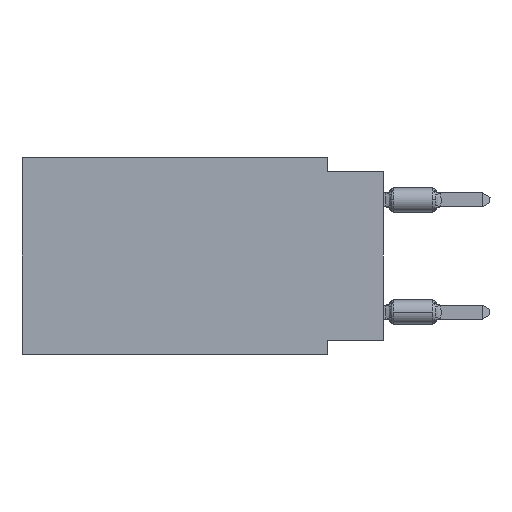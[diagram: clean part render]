
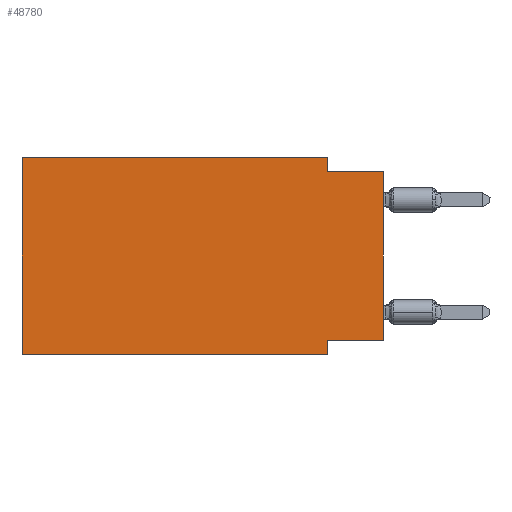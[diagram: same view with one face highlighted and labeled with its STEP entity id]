
A CAD part, left-side view. The second image highlights one B-rep face of the part: STEP entity #48780.
In plain terms, the highlighted planar face has unit normal (-1, 0, 0).
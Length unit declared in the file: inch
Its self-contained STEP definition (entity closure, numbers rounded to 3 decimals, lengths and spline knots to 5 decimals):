
#2103 = LINE ( 'NONE', #14832, #36640 ) ;
#2127 = EDGE_LOOP ( 'NONE', ( #13513, #40469, #35903, #5322, #4521, #36435, #36315, #18551 ) ) ;
#4039 = CARTESIAN_POINT ( 'NONE',  ( 0., 0.645, -0.35 ) ) ;
#4342 = FACE_OUTER_BOUND ( 'NONE', #2127, .T. ) ;
#4521 = ORIENTED_EDGE ( 'NONE', *, *, #28124, .F. ) ;
#5254 = CARTESIAN_POINT ( 'NONE',  ( 0., 0.1, -0.025 ) ) ;
#5322 = ORIENTED_EDGE ( 'NONE', *, *, #10600, .F. ) ;
#5991 = CARTESIAN_POINT ( 'NONE',  ( 0., 0.1, -0.35 ) ) ;
#7587 = LINE ( 'NONE', #23304, #27997 ) ;
#7668 = DIRECTION ( 'NONE',  ( 0., 0., -1. ) ) ;
#7987 = VERTEX_POINT ( 'NONE', #14603 ) ;
#10600 = EDGE_CURVE ( 'NONE', #7987, #50869, #49527, .T. ) ;
#10712 = EDGE_CURVE ( 'NONE', #32661, #44551, #46809, .T. ) ;
#11478 = CARTESIAN_POINT ( 'NONE',  ( 0., 0.1, -0.325 ) ) ;
#12235 = CARTESIAN_POINT ( 'NONE',  ( 0., 0.645, 0. ) ) ;
#13513 = ORIENTED_EDGE ( 'NONE', *, *, #34205, .T. ) ;
#14603 = CARTESIAN_POINT ( 'NONE',  ( 0., 0.645, 0. ) ) ;
#14832 = CARTESIAN_POINT ( 'NONE',  ( 0., 0.645, 0. ) ) ;
#16035 = EDGE_CURVE ( 'NONE', #44551, #33848, #43034, .T. ) ;
#16199 = AXIS2_PLACEMENT_3D ( 'NONE', #50549, #38377, #45419 ) ;
#16361 = VECTOR ( 'NONE', #24399, 39.37008 ) ;
#18551 = ORIENTED_EDGE ( 'NONE', *, *, #10712, .F. ) ;
#19239 = CARTESIAN_POINT ( 'NONE',  ( 0., 0., 0. ) ) ;
#20438 = CARTESIAN_POINT ( 'NONE',  ( 0., 0., -0.325 ) ) ;
#21376 = VERTEX_POINT ( 'NONE', #5254 ) ;
#22820 = CARTESIAN_POINT ( 'NONE',  ( 0., 0., -0.025 ) ) ;
#22997 = VECTOR ( 'NONE', #50339, 39.37008 ) ;
#23304 = CARTESIAN_POINT ( 'NONE',  ( 0., 0.645, -0.35 ) ) ;
#24399 = DIRECTION ( 'NONE',  ( 0., -1., 0. ) ) ;
#24421 = LINE ( 'NONE', #39720, #49111 ) ;
#24472 = VECTOR ( 'NONE', #7668, 39.37008 ) ;
#24663 = EDGE_CURVE ( 'NONE', #50869, #21376, #40655, .T. ) ;
#25563 = CARTESIAN_POINT ( 'NONE',  ( 0., 0.1, -0.35 ) ) ;
#26189 = DIRECTION ( 'NONE',  ( 0., 0., 1. ) ) ;
#27438 = VECTOR ( 'NONE', #28402, 39.37008 ) ;
#27997 = VECTOR ( 'NONE', #52208, 39.37008 ) ;
#28124 = EDGE_CURVE ( 'NONE', #50912, #7987, #2103, .T. ) ;
#28402 = DIRECTION ( 'NONE',  ( 0., 0., 1. ) ) ;
#32661 = VERTEX_POINT ( 'NONE', #20438 ) ;
#33848 = VERTEX_POINT ( 'NONE', #25563 ) ;
#34205 = EDGE_CURVE ( 'NONE', #32661, #48083, #35963, .T. ) ;
#35599 = EDGE_CURVE ( 'NONE', #21376, #48083, #24421, .T. ) ;
#35903 = ORIENTED_EDGE ( 'NONE', *, *, #24663, .F. ) ;
#35963 = LINE ( 'NONE', #19239, #27438 ) ;
#36315 = ORIENTED_EDGE ( 'NONE', *, *, #16035, .F. ) ;
#36435 = ORIENTED_EDGE ( 'NONE', *, *, #43540, .T. ) ;
#36640 = VECTOR ( 'NONE', #26189, 39.37008 ) ;
#38377 = DIRECTION ( 'NONE',  ( 1., 0., 0. ) ) ;
#39720 = CARTESIAN_POINT ( 'NONE',  ( 0., 0., -0.025 ) ) ;
#40388 = CARTESIAN_POINT ( 'NONE',  ( 0., 0.1, 0. ) ) ;
#40469 = ORIENTED_EDGE ( 'NONE', *, *, #35599, .F. ) ;
#40655 = LINE ( 'NONE', #40388, #24472 ) ;
#41641 = PLANE ( 'NONE',  #16199 ) ;
#42231 = DIRECTION ( 'NONE',  ( 0., 1., 0. ) ) ;
#42502 = CARTESIAN_POINT ( 'NONE',  ( 0., 0., -0.325 ) ) ;
#42553 = CARTESIAN_POINT ( 'NONE',  ( 0., 0.1, 0. ) ) ;
#43034 = LINE ( 'NONE', #5991, #22997 ) ;
#43540 = EDGE_CURVE ( 'NONE', #50912, #33848, #7587, .T. ) ;
#44005 = VECTOR ( 'NONE', #42231, 39.37008 ) ;
#44551 = VERTEX_POINT ( 'NONE', #11478 ) ;
#45419 = DIRECTION ( 'NONE',  ( 0., 0., -1. ) ) ;
#46809 = LINE ( 'NONE', #42502, #44005 ) ;
#48083 = VERTEX_POINT ( 'NONE', #22820 ) ;
#48780 = ADVANCED_FACE ( 'NONE', ( #4342 ), #41641, .F. ) ;
#49111 = VECTOR ( 'NONE', #51091, 39.37008 ) ;
#49527 = LINE ( 'NONE', #12235, #16361 ) ;
#50339 = DIRECTION ( 'NONE',  ( 0., 0., -1. ) ) ;
#50549 = CARTESIAN_POINT ( 'NONE',  ( 0., 0.645, 0. ) ) ;
#50869 = VERTEX_POINT ( 'NONE', #42553 ) ;
#50912 = VERTEX_POINT ( 'NONE', #4039 ) ;
#51091 = DIRECTION ( 'NONE',  ( 0., -1., 0. ) ) ;
#52208 = DIRECTION ( 'NONE',  ( 0., -1., 0. ) ) ;
